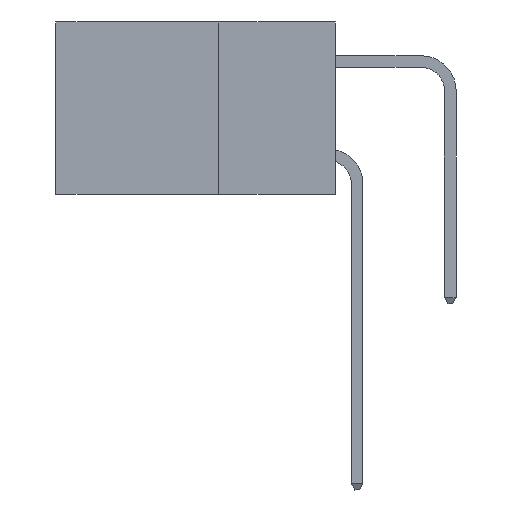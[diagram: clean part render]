
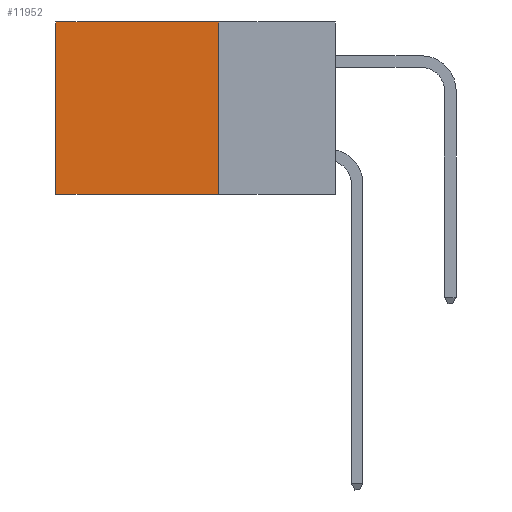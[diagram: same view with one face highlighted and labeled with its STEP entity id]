
A CAD part, left-side view. The second image highlights one B-rep face of the part: STEP entity #11952.
In plain terms, the highlighted planar face has unit normal (-1, 0, 0).
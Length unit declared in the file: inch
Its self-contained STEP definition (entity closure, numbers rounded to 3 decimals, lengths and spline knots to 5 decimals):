
#2061 = DIRECTION ( 'NONE',  ( 0., 1., 0. ) ) ;
#2835 = FACE_OUTER_BOUND ( 'NONE', #33756, .T. ) ;
#2912 = ORIENTED_EDGE ( 'NONE', *, *, #5774, .F. ) ;
#3283 = PLANE ( 'NONE',  #30380 ) ;
#3457 = VERTEX_POINT ( 'NONE', #28886 ) ;
#4928 = CARTESIAN_POINT ( 'NONE',  ( 0.2875, 0.25, 0. ) ) ;
#5774 = EDGE_CURVE ( 'NONE', #39784, #3457, #37289, .T. ) ;
#6600 = DIRECTION ( 'NONE',  ( 0., 1., 0. ) ) ;
#7425 = ORIENTED_EDGE ( 'NONE', *, *, #37265, .T. ) ;
#8711 = ORIENTED_EDGE ( 'NONE', *, *, #38949, .F. ) ;
#8903 = CARTESIAN_POINT ( 'NONE',  ( 0.2875, 0.25, -0.37 ) ) ;
#8944 = DIRECTION ( 'NONE',  ( 0., 0., -1. ) ) ;
#10260 = DIRECTION ( 'NONE',  ( 0., 0., -1. ) ) ;
#10561 = VECTOR ( 'NONE', #19102, 39.37008 ) ;
#11952 = ADVANCED_FACE ( 'NONE', ( #2835 ), #3283, .F. ) ;
#13910 = LINE ( 'NONE', #26881, #29622 ) ;
#14861 = VECTOR ( 'NONE', #8944, 39.37008 ) ;
#15697 = CARTESIAN_POINT ( 'NONE',  ( 0.2875, 0.25, 0. ) ) ;
#16988 = LINE ( 'NONE', #39278, #14861 ) ;
#19102 = DIRECTION ( 'NONE',  ( 0., 0., -1. ) ) ;
#23436 = VERTEX_POINT ( 'NONE', #35147 ) ;
#26341 = CARTESIAN_POINT ( 'NONE',  ( 0.2875, 0.6, -0.37 ) ) ;
#26881 = CARTESIAN_POINT ( 'NONE',  ( 0.2875, 0.25, 0. ) ) ;
#27045 = CARTESIAN_POINT ( 'NONE',  ( 0.2875, 0.25, 0. ) ) ;
#28886 = CARTESIAN_POINT ( 'NONE',  ( 0.2875, 0.25, -0.37 ) ) ;
#29179 = ORIENTED_EDGE ( 'NONE', *, *, #41076, .T. ) ;
#29622 = VECTOR ( 'NONE', #6600, 39.37008 ) ;
#30380 = AXIS2_PLACEMENT_3D ( 'NONE', #27045, #30422, #10260 ) ;
#30422 = DIRECTION ( 'NONE',  ( 1., 0., 0. ) ) ;
#33615 = LINE ( 'NONE', #8903, #41387 ) ;
#33756 = EDGE_LOOP ( 'NONE', ( #29179, #8711, #2912, #7425 ) ) ;
#34143 = VERTEX_POINT ( 'NONE', #26341 ) ;
#35147 = CARTESIAN_POINT ( 'NONE',  ( 0.2875, 0.6, 0. ) ) ;
#37265 = EDGE_CURVE ( 'NONE', #39784, #23436, #13910, .T. ) ;
#37289 = LINE ( 'NONE', #15697, #10561 ) ;
#38949 = EDGE_CURVE ( 'NONE', #3457, #34143, #33615, .T. ) ;
#39278 = CARTESIAN_POINT ( 'NONE',  ( 0.2875, 0.6, 0. ) ) ;
#39784 = VERTEX_POINT ( 'NONE', #4928 ) ;
#41076 = EDGE_CURVE ( 'NONE', #23436, #34143, #16988, .T. ) ;
#41387 = VECTOR ( 'NONE', #2061, 39.37008 ) ;
